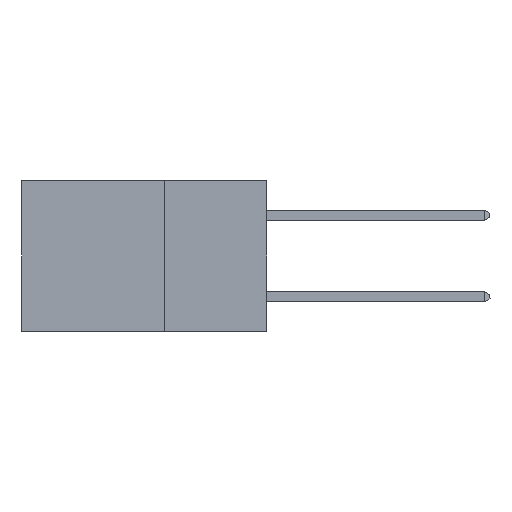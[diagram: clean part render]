
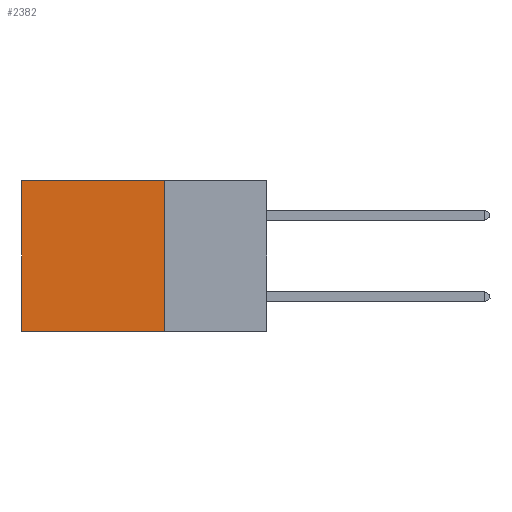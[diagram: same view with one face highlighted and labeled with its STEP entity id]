
A CAD part, left-side view. The second image highlights one B-rep face of the part: STEP entity #2382.
In plain terms, the highlighted planar face has unit normal (-1, 0, 0).
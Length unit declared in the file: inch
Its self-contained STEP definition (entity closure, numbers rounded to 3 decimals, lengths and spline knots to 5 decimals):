
#1151 = EDGE_CURVE ( 'NONE', #15071, #12118, #16809, .T. ) ;
#1189 = ORIENTED_EDGE ( 'NONE', *, *, #1151, .T. ) ;
#1395 = ORIENTED_EDGE ( 'NONE', *, *, #16832, .T. ) ;
#1625 = VECTOR ( 'NONE', #7568, 39.37008 ) ;
#1669 = ORIENTED_EDGE ( 'NONE', *, *, #9589, .F. ) ;
#2350 = VECTOR ( 'NONE', #15458, 39.37008 ) ;
#2382 = ADVANCED_FACE ( 'NONE', ( #10929 ), #17562, .F. ) ;
#3152 = CARTESIAN_POINT ( 'NONE',  ( 0.2875, 0.25, -0.37 ) ) ;
#5097 = ORIENTED_EDGE ( 'NONE', *, *, #6789, .F. ) ;
#6006 = CARTESIAN_POINT ( 'NONE',  ( 0.2875, 0.25, 0. ) ) ;
#6106 = LINE ( 'NONE', #3152, #2350 ) ;
#6188 = LINE ( 'NONE', #6006, #9145 ) ;
#6789 = EDGE_CURVE ( 'NONE', #11981, #12118, #6106, .T. ) ;
#6961 = CARTESIAN_POINT ( 'NONE',  ( 0.2875, 0.25, -0.37 ) ) ;
#7568 = DIRECTION ( 'NONE',  ( 0., 0., -1. ) ) ;
#7675 = CARTESIAN_POINT ( 'NONE',  ( 0.2875, 0.6, 0. ) ) ;
#8021 = VERTEX_POINT ( 'NONE', #11050 ) ;
#8335 = VECTOR ( 'NONE', #17321, 39.37008 ) ;
#8788 = LINE ( 'NONE', #15972, #8335 ) ;
#9145 = VECTOR ( 'NONE', #10279, 39.37008 ) ;
#9589 = EDGE_CURVE ( 'NONE', #8021, #11981, #8788, .T. ) ;
#10061 = EDGE_LOOP ( 'NONE', ( #1189, #5097, #1669, #1395 ) ) ;
#10279 = DIRECTION ( 'NONE',  ( 0., 1., 0. ) ) ;
#10929 = FACE_OUTER_BOUND ( 'NONE', #10061, .T. ) ;
#11050 = CARTESIAN_POINT ( 'NONE',  ( 0.2875, 0.25, 0. ) ) ;
#11981 = VERTEX_POINT ( 'NONE', #6961 ) ;
#12118 = VERTEX_POINT ( 'NONE', #17897 ) ;
#13262 = AXIS2_PLACEMENT_3D ( 'NONE', #17797, #17539, #17503 ) ;
#15071 = VERTEX_POINT ( 'NONE', #7675 ) ;
#15458 = DIRECTION ( 'NONE',  ( 0., 1., 0. ) ) ;
#15972 = CARTESIAN_POINT ( 'NONE',  ( 0.2875, 0.25, 0. ) ) ;
#16389 = CARTESIAN_POINT ( 'NONE',  ( 0.2875, 0.6, 0. ) ) ;
#16809 = LINE ( 'NONE', #16389, #1625 ) ;
#16832 = EDGE_CURVE ( 'NONE', #8021, #15071, #6188, .T. ) ;
#17321 = DIRECTION ( 'NONE',  ( 0., 0., -1. ) ) ;
#17503 = DIRECTION ( 'NONE',  ( 0., 0., -1. ) ) ;
#17539 = DIRECTION ( 'NONE',  ( 1., 0., 0. ) ) ;
#17562 = PLANE ( 'NONE',  #13262 ) ;
#17797 = CARTESIAN_POINT ( 'NONE',  ( 0.2875, 0.25, 0. ) ) ;
#17897 = CARTESIAN_POINT ( 'NONE',  ( 0.2875, 0.6, -0.37 ) ) ;
